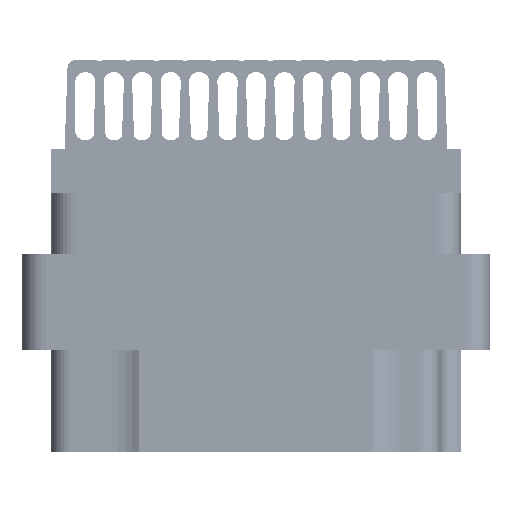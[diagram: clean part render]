
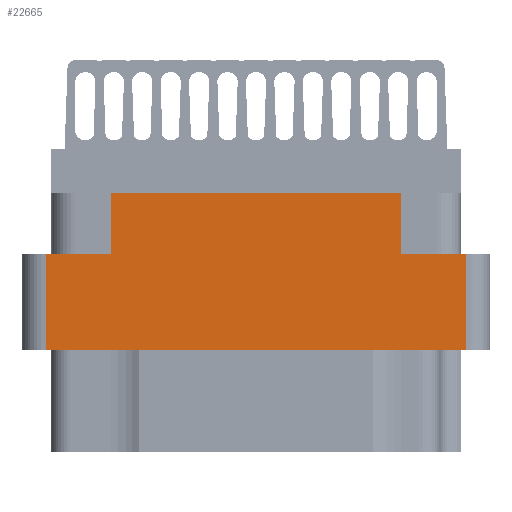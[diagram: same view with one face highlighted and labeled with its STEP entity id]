
A CAD part, left-side view. The second image highlights one B-rep face of the part: STEP entity #22665.
In plain terms, the highlighted planar face has unit normal (-1, 0, 0).
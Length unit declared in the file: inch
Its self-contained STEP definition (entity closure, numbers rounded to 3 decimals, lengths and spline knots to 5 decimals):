
#45 = DIRECTION ( 'NONE',  ( 0., 0., 1. ) ) ;
#614 = CARTESIAN_POINT ( 'NONE',  ( -1.359, 0.555, -0.277 ) ) ;
#2918 = ORIENTED_EDGE ( 'NONE', *, *, #73069, .F. ) ;
#3669 = DIRECTION ( 'NONE',  ( 0., -1., 0. ) ) ;
#4017 = LINE ( 'NONE', #20668, #37085 ) ;
#4101 = CARTESIAN_POINT ( 'NONE',  ( -1.359, 0., -0.277 ) ) ;
#6537 = ORIENTED_EDGE ( 'NONE', *, *, #60457, .T. ) ;
#9678 = LINE ( 'NONE', #64782, #74212 ) ;
#10894 = VERTEX_POINT ( 'NONE', #23011 ) ;
#10932 = CARTESIAN_POINT ( 'NONE',  ( -1.359, -0.3825, -0.117 ) ) ;
#12293 = ORIENTED_EDGE ( 'NONE', *, *, #32120, .T. ) ;
#13706 = VECTOR ( 'NONE', #45, 39.37008 ) ;
#15193 = DIRECTION ( 'NONE',  ( 0., 0., 1. ) ) ;
#15455 = CARTESIAN_POINT ( 'NONE',  ( -1.359, -0.555, -0.798 ) ) ;
#17067 = VERTEX_POINT ( 'NONE', #19647 ) ;
#19647 = CARTESIAN_POINT ( 'NONE',  ( -1.359, -0.555, -0.277 ) ) ;
#20668 = CARTESIAN_POINT ( 'NONE',  ( -1.359, 0.617, -0.117 ) ) ;
#20851 = DIRECTION ( 'NONE',  ( 0., -1., 0. ) ) ;
#22424 = LINE ( 'NONE', #57957, #26002 ) ;
#22632 = VERTEX_POINT ( 'NONE', #10932 ) ;
#22665 = ADVANCED_FACE ( 'NONE', ( #54234 ), #35417, .T. ) ;
#22992 = EDGE_CURVE ( 'NONE', #73428, #30580, #33551, .T. ) ;
#23011 = CARTESIAN_POINT ( 'NONE',  ( -1.359, -0.555, -0.529 ) ) ;
#23593 = DIRECTION ( 'NONE',  ( 0., 0., -1. ) ) ;
#26002 = VECTOR ( 'NONE', #23593, 39.37008 ) ;
#26174 = CARTESIAN_POINT ( 'NONE',  ( -1.359, 0.555, -0.529 ) ) ;
#26344 = EDGE_CURVE ( 'NONE', #30580, #72287, #28900, .T. ) ;
#28900 = LINE ( 'NONE', #34364, #13706 ) ;
#29412 = DIRECTION ( 'NONE',  ( 0., 0., 1. ) ) ;
#29915 = CARTESIAN_POINT ( 'NONE',  ( -1.359, -0.617, -0.798 ) ) ;
#29997 = EDGE_LOOP ( 'NONE', ( #72432, #6537, #65608, #12293, #52853, #47759, #2918, #31482 ) ) ;
#30580 = VERTEX_POINT ( 'NONE', #58754 ) ;
#31482 = ORIENTED_EDGE ( 'NONE', *, *, #26344, .F. ) ;
#32082 = LINE ( 'NONE', #67329, #66167 ) ;
#32120 = EDGE_CURVE ( 'NONE', #10894, #17067, #65395, .T. ) ;
#33551 = LINE ( 'NONE', #4101, #38943 ) ;
#34364 = CARTESIAN_POINT ( 'NONE',  ( -1.359, 0.3825, -0.277 ) ) ;
#34907 = VECTOR ( 'NONE', #15193, 39.37008 ) ;
#34998 = EDGE_CURVE ( 'NONE', #10894, #55377, #40765, .T. ) ;
#35417 = PLANE ( 'NONE',  #60878 ) ;
#35571 = CARTESIAN_POINT ( 'NONE',  ( -1.359, -0.3825, -0.277 ) ) ;
#37085 = VECTOR ( 'NONE', #3669, 39.37008 ) ;
#38943 = VECTOR ( 'NONE', #20851, 39.37008 ) ;
#40765 = LINE ( 'NONE', #63450, #73892 ) ;
#45875 = DIRECTION ( 'NONE',  ( 0., 1., 0. ) ) ;
#47308 = VERTEX_POINT ( 'NONE', #35571 ) ;
#47759 = ORIENTED_EDGE ( 'NONE', *, *, #56636, .T. ) ;
#50043 = DIRECTION ( 'NONE',  ( 0., 0., 1. ) ) ;
#52853 = ORIENTED_EDGE ( 'NONE', *, *, #66627, .F. ) ;
#54234 = FACE_OUTER_BOUND ( 'NONE', #29997, .T. ) ;
#54707 = DIRECTION ( 'NONE',  ( 0., -1., 0. ) ) ;
#54856 = CARTESIAN_POINT ( 'NONE',  ( -1.359, 0.3825, -0.117 ) ) ;
#55377 = VERTEX_POINT ( 'NONE', #26174 ) ;
#56636 = EDGE_CURVE ( 'NONE', #47308, #22632, #32082, .T. ) ;
#57957 = CARTESIAN_POINT ( 'NONE',  ( -1.359, 0.555, -0.798 ) ) ;
#58754 = CARTESIAN_POINT ( 'NONE',  ( -1.359, 0.3825, -0.277 ) ) ;
#60457 = EDGE_CURVE ( 'NONE', #73428, #55377, #22424, .T. ) ;
#60878 = AXIS2_PLACEMENT_3D ( 'NONE', #29915, #63789, #29412 ) ;
#63450 = CARTESIAN_POINT ( 'NONE',  ( -1.359, 0., -0.529 ) ) ;
#63789 = DIRECTION ( 'NONE',  ( -1., 0., 0. ) ) ;
#64782 = CARTESIAN_POINT ( 'NONE',  ( -1.359, 0., -0.277 ) ) ;
#65395 = LINE ( 'NONE', #15455, #34907 ) ;
#65608 = ORIENTED_EDGE ( 'NONE', *, *, #34998, .F. ) ;
#66167 = VECTOR ( 'NONE', #50043, 39.37008 ) ;
#66627 = EDGE_CURVE ( 'NONE', #47308, #17067, #9678, .T. ) ;
#67329 = CARTESIAN_POINT ( 'NONE',  ( -1.359, -0.3825, -0.277 ) ) ;
#72287 = VERTEX_POINT ( 'NONE', #54856 ) ;
#72432 = ORIENTED_EDGE ( 'NONE', *, *, #22992, .F. ) ;
#73069 = EDGE_CURVE ( 'NONE', #72287, #22632, #4017, .T. ) ;
#73428 = VERTEX_POINT ( 'NONE', #614 ) ;
#73892 = VECTOR ( 'NONE', #45875, 39.37008 ) ;
#74212 = VECTOR ( 'NONE', #54707, 39.37008 ) ;
